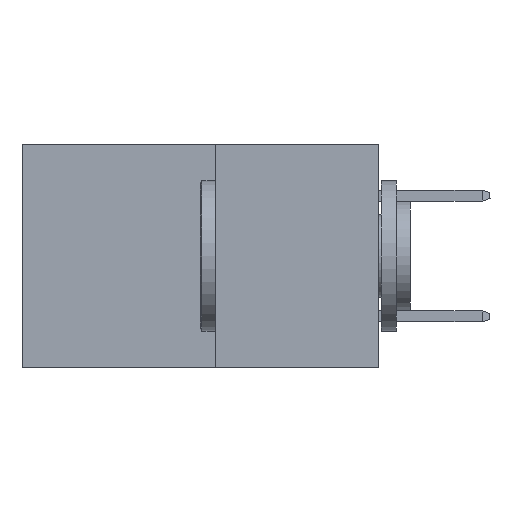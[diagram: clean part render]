
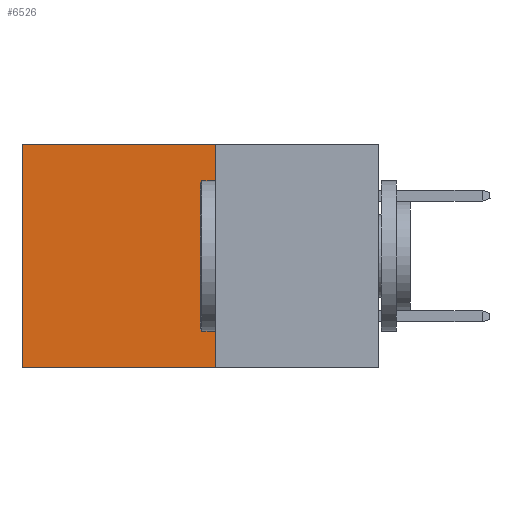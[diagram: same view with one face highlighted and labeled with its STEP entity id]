
A CAD part, left-side view. The second image highlights one B-rep face of the part: STEP entity #6526.
In plain terms, the highlighted planar face has unit normal (-1, 0, 0).
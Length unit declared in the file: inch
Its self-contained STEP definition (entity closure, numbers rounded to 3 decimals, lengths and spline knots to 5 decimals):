
#580 = VERTEX_POINT ( 'NONE', #5771 ) ;
#1181 = CARTESIAN_POINT ( 'NONE',  ( 0.277, 0.59, -0.37 ) ) ;
#2355 = CARTESIAN_POINT ( 'NONE',  ( 0.277, 0.27, 0. ) ) ;
#3138 = ORIENTED_EDGE ( 'NONE', *, *, #3743, .T. ) ;
#3230 = CARTESIAN_POINT ( 'NONE',  ( 0.277, 0.27, -0.37 ) ) ;
#3743 = EDGE_CURVE ( 'NONE', #580, #14797, #5417, .T. ) ;
#4404 = DIRECTION ( 'NONE',  ( 0., 1., 0. ) ) ;
#4807 = LINE ( 'NONE', #8329, #10640 ) ;
#5053 = VECTOR ( 'NONE', #11493, 39.37008 ) ;
#5352 = ORIENTED_EDGE ( 'NONE', *, *, #9048, .F. ) ;
#5401 = AXIS2_PLACEMENT_3D ( 'NONE', #14168, #12748, #9908 ) ;
#5417 = LINE ( 'NONE', #1181, #5053 ) ;
#5678 = CARTESIAN_POINT ( 'NONE',  ( 0.277, 0.59, -0.37 ) ) ;
#5771 = CARTESIAN_POINT ( 'NONE',  ( 0.277, 0.59, 0. ) ) ;
#5795 = ORIENTED_EDGE ( 'NONE', *, *, #7894, .T. ) ;
#6235 = VECTOR ( 'NONE', #8900, 39.37008 ) ;
#6526 = ADVANCED_FACE ( 'NONE', ( #8391 ), #6824, .F. ) ;
#6824 = PLANE ( 'NONE',  #5401 ) ;
#7073 = CARTESIAN_POINT ( 'NONE',  ( 0.277, 0.27, -0.37 ) ) ;
#7315 = ORIENTED_EDGE ( 'NONE', *, *, #11641, .F. ) ;
#7894 = EDGE_CURVE ( 'NONE', #12154, #580, #9666, .T. ) ;
#8329 = CARTESIAN_POINT ( 'NONE',  ( 0.277, 0.27, -0.37 ) ) ;
#8391 = FACE_OUTER_BOUND ( 'NONE', #12327, .T. ) ;
#8900 = DIRECTION ( 'NONE',  ( 0., 1., 0. ) ) ;
#9048 = EDGE_CURVE ( 'NONE', #13390, #14797, #13272, .T. ) ;
#9516 = DIRECTION ( 'NONE',  ( 0., 0., -1. ) ) ;
#9666 = LINE ( 'NONE', #9871, #6235 ) ;
#9871 = CARTESIAN_POINT ( 'NONE',  ( 0.277, 0.27, 0. ) ) ;
#9908 = DIRECTION ( 'NONE',  ( 0., 0., -1. ) ) ;
#10640 = VECTOR ( 'NONE', #9516, 39.37008 ) ;
#11493 = DIRECTION ( 'NONE',  ( 0., 0., -1. ) ) ;
#11641 = EDGE_CURVE ( 'NONE', #12154, #13390, #4807, .T. ) ;
#12154 = VERTEX_POINT ( 'NONE', #2355 ) ;
#12327 = EDGE_LOOP ( 'NONE', ( #3138, #5352, #7315, #5795 ) ) ;
#12748 = DIRECTION ( 'NONE',  ( 1., 0., 0. ) ) ;
#13272 = LINE ( 'NONE', #3230, #15168 ) ;
#13390 = VERTEX_POINT ( 'NONE', #7073 ) ;
#14168 = CARTESIAN_POINT ( 'NONE',  ( 0.277, 0.27, -0.37 ) ) ;
#14797 = VERTEX_POINT ( 'NONE', #5678 ) ;
#15168 = VECTOR ( 'NONE', #4404, 39.37008 ) ;
